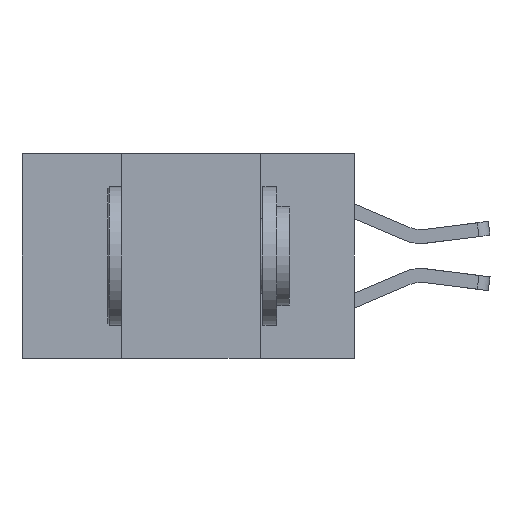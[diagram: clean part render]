
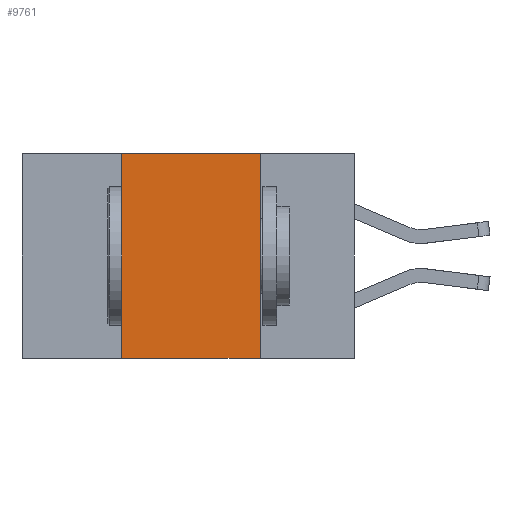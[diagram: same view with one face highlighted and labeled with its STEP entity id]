
A CAD part, left-side view. The second image highlights one B-rep face of the part: STEP entity #9761.
In plain terms, the highlighted planar face has unit normal (-1, 0, 0).
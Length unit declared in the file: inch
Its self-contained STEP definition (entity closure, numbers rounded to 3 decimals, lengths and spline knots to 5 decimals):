
#114 = CARTESIAN_POINT ( 'NONE',  ( 0., 0.6, 0. ) ) ;
#136 = FACE_OUTER_BOUND ( 'NONE', #4714, .T. ) ;
#355 = LINE ( 'NONE', #10426, #6626 ) ;
#611 = EDGE_CURVE ( 'NONE', #8121, #7257, #3011, .T. ) ;
#1475 = CARTESIAN_POINT ( 'NONE',  ( 0., 0.17, 0. ) ) ;
#1739 = DIRECTION ( 'NONE',  ( 0., -1., 0. ) ) ;
#1781 = ORIENTED_EDGE ( 'NONE', *, *, #6038, .F. ) ;
#1925 = VERTEX_POINT ( 'NONE', #8306 ) ;
#2198 = CARTESIAN_POINT ( 'NONE',  ( 0., 0.17, -0.37 ) ) ;
#2446 = ORIENTED_EDGE ( 'NONE', *, *, #611, .F. ) ;
#2525 = VECTOR ( 'NONE', #7093, 39.37008 ) ;
#2646 = DIRECTION ( 'NONE',  ( 1., 0., 0. ) ) ;
#3011 = LINE ( 'NONE', #1475, #2525 ) ;
#3087 = AXIS2_PLACEMENT_3D ( 'NONE', #3353, #2646, #4990 ) ;
#3126 = ORIENTED_EDGE ( 'NONE', *, *, #4017, .F. ) ;
#3353 = CARTESIAN_POINT ( 'NONE',  ( 0., 0.6, 0. ) ) ;
#3356 = VERTEX_POINT ( 'NONE', #9829 ) ;
#4017 = EDGE_CURVE ( 'NONE', #3356, #1925, #4643, .T. ) ;
#4105 = DIRECTION ( 'NONE',  ( 0., -1., 0. ) ) ;
#4220 = PLANE ( 'NONE',  #3087 ) ;
#4643 = LINE ( 'NONE', #5620, #5550 ) ;
#4714 = EDGE_LOOP ( 'NONE', ( #2446, #1781, #3126, #9751 ) ) ;
#4990 = DIRECTION ( 'NONE',  ( 0., 0., -1. ) ) ;
#5550 = VECTOR ( 'NONE', #8088, 39.37008 ) ;
#5620 = CARTESIAN_POINT ( 'NONE',  ( 0., 0.42, 0. ) ) ;
#6038 = EDGE_CURVE ( 'NONE', #1925, #8121, #7027, .T. ) ;
#6363 = EDGE_CURVE ( 'NONE', #3356, #7257, #355, .T. ) ;
#6626 = VECTOR ( 'NONE', #4105, 39.37008 ) ;
#7027 = LINE ( 'NONE', #114, #10188 ) ;
#7093 = DIRECTION ( 'NONE',  ( 0., 0., -1. ) ) ;
#7257 = VERTEX_POINT ( 'NONE', #2198 ) ;
#8088 = DIRECTION ( 'NONE',  ( 0., 0., 1. ) ) ;
#8121 = VERTEX_POINT ( 'NONE', #9526 ) ;
#8306 = CARTESIAN_POINT ( 'NONE',  ( 0., 0.42, 0. ) ) ;
#9526 = CARTESIAN_POINT ( 'NONE',  ( 0., 0.17, 0. ) ) ;
#9751 = ORIENTED_EDGE ( 'NONE', *, *, #6363, .T. ) ;
#9761 = ADVANCED_FACE ( 'NONE', ( #136 ), #4220, .F. ) ;
#9829 = CARTESIAN_POINT ( 'NONE',  ( 0., 0.42, -0.37 ) ) ;
#10188 = VECTOR ( 'NONE', #1739, 39.37008 ) ;
#10426 = CARTESIAN_POINT ( 'NONE',  ( 0., 0.6, -0.37 ) ) ;
